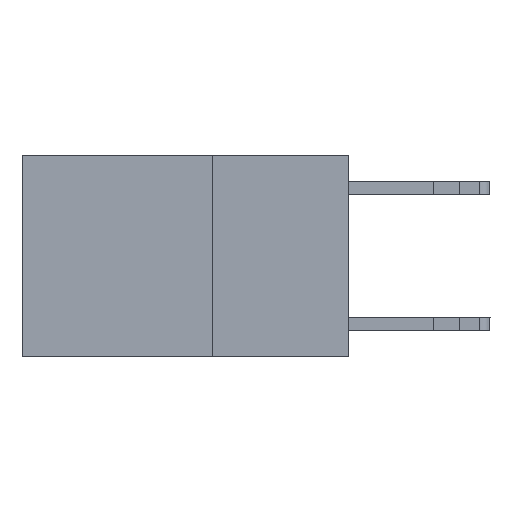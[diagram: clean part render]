
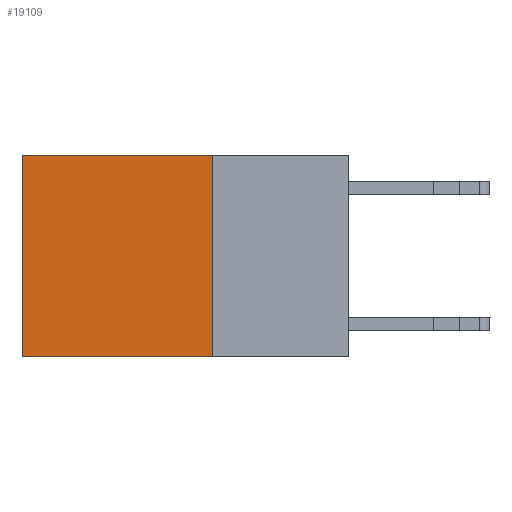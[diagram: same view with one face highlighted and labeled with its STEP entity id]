
A CAD part, left-side view. The second image highlights one B-rep face of the part: STEP entity #19109.
In plain terms, the highlighted planar face has unit normal (-1, 0, 0).
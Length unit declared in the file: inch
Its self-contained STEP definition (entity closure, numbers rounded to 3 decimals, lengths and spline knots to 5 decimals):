
#246 = CARTESIAN_POINT ( 'NONE',  ( 0.2625, 0.6, -0.37 ) ) ;
#888 = VECTOR ( 'NONE', #19242, 39.37008 ) ;
#1258 = VERTEX_POINT ( 'NONE', #5299 ) ;
#1653 = LINE ( 'NONE', #17104, #888 ) ;
#2431 = VERTEX_POINT ( 'NONE', #3383 ) ;
#3383 = CARTESIAN_POINT ( 'NONE',  ( 0.2625, 0.25, 0. ) ) ;
#3400 = EDGE_CURVE ( 'NONE', #17294, #18638, #8034, .T. ) ;
#3756 = EDGE_CURVE ( 'NONE', #2431, #1258, #1653, .T. ) ;
#5299 = CARTESIAN_POINT ( 'NONE',  ( 0.2625, 0.25, -0.37 ) ) ;
#7146 = EDGE_CURVE ( 'NONE', #2431, #17294, #21824, .T. ) ;
#7231 = VECTOR ( 'NONE', #16552, 39.37008 ) ;
#7437 = ORIENTED_EDGE ( 'NONE', *, *, #7146, .T. ) ;
#7497 = EDGE_LOOP ( 'NONE', ( #23678, #22391, #13804, #7437 ) ) ;
#8034 = LINE ( 'NONE', #16409, #7231 ) ;
#9205 = DIRECTION ( 'NONE',  ( 1., 0., 0. ) ) ;
#10521 = LINE ( 'NONE', #20607, #19773 ) ;
#12380 = FACE_OUTER_BOUND ( 'NONE', #7497, .T. ) ;
#13804 = ORIENTED_EDGE ( 'NONE', *, *, #3756, .F. ) ;
#14670 = EDGE_CURVE ( 'NONE', #1258, #18638, #10521, .T. ) ;
#16409 = CARTESIAN_POINT ( 'NONE',  ( 0.2625, 0.6, 0. ) ) ;
#16552 = DIRECTION ( 'NONE',  ( 0., 0., -1. ) ) ;
#17104 = CARTESIAN_POINT ( 'NONE',  ( 0.2625, 0.25, 0. ) ) ;
#17294 = VERTEX_POINT ( 'NONE', #22290 ) ;
#18377 = PLANE ( 'NONE',  #18678 ) ;
#18638 = VERTEX_POINT ( 'NONE', #246 ) ;
#18678 = AXIS2_PLACEMENT_3D ( 'NONE', #21970, #9205, #22039 ) ;
#19109 = ADVANCED_FACE ( 'NONE', ( #12380 ), #18377, .F. ) ;
#19242 = DIRECTION ( 'NONE',  ( 0., 0., -1. ) ) ;
#19773 = VECTOR ( 'NONE', #20526, 39.37008 ) ;
#20526 = DIRECTION ( 'NONE',  ( 0., 1., 0. ) ) ;
#20607 = CARTESIAN_POINT ( 'NONE',  ( 0.2625, 0.25, -0.37 ) ) ;
#20835 = DIRECTION ( 'NONE',  ( 0., 1., 0. ) ) ;
#20950 = CARTESIAN_POINT ( 'NONE',  ( 0.2625, 0.25, 0. ) ) ;
#21700 = VECTOR ( 'NONE', #20835, 39.37008 ) ;
#21824 = LINE ( 'NONE', #20950, #21700 ) ;
#21970 = CARTESIAN_POINT ( 'NONE',  ( 0.2625, 0.25, 0. ) ) ;
#22039 = DIRECTION ( 'NONE',  ( 0., 0., -1. ) ) ;
#22290 = CARTESIAN_POINT ( 'NONE',  ( 0.2625, 0.6, 0. ) ) ;
#22391 = ORIENTED_EDGE ( 'NONE', *, *, #14670, .F. ) ;
#23678 = ORIENTED_EDGE ( 'NONE', *, *, #3400, .T. ) ;
